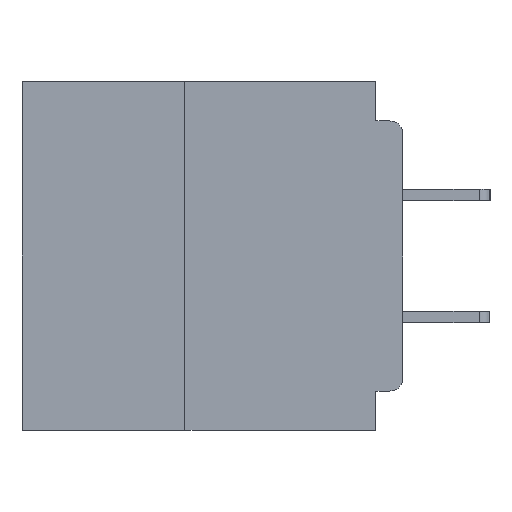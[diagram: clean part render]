
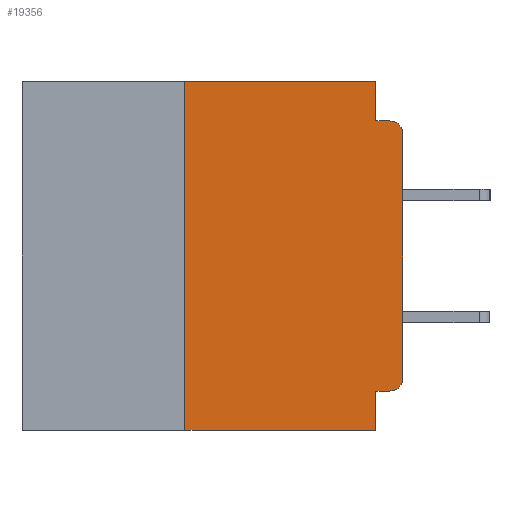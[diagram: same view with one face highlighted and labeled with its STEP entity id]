
A CAD part, left-side view. The second image highlights one B-rep face of the part: STEP entity #19356.
In plain terms, the highlighted planar face has unit normal (-1, 0, 0).
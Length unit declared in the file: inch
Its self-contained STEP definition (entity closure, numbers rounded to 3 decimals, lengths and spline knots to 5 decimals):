
#174 = ORIENTED_EDGE ( 'NONE', *, *, #10337, .T. ) ;
#470 = EDGE_CURVE ( 'NONE', #36528, #20524, #12697, .T. ) ;
#1134 = CARTESIAN_POINT ( 'NONE',  ( 0., 0.015, -0.045 ) ) ;
#1625 = CARTESIAN_POINT ( 'NONE',  ( 0., 0.031, -0.045 ) ) ;
#1760 = CARTESIAN_POINT ( 'NONE',  ( 0., 0.031, -0.355 ) ) ;
#1807 = FACE_OUTER_BOUND ( 'NONE', #8016, .T. ) ;
#3209 = CARTESIAN_POINT ( 'NONE',  ( 0., 0.031, 0. ) ) ;
#5400 = ORIENTED_EDGE ( 'NONE', *, *, #17535, .T. ) ;
#6367 = CARTESIAN_POINT ( 'NONE',  ( 0., 0.031, 0. ) ) ;
#7665 = CARTESIAN_POINT ( 'NONE',  ( 0., 0., -0.355 ) ) ;
#7924 = LINE ( 'NONE', #15533, #16364 ) ;
#8009 = VERTEX_POINT ( 'NONE', #31164 ) ;
#8016 = EDGE_LOOP ( 'NONE', ( #5400, #14799, #31670, #36529, #31976, #8084, #174, #28848, #18778, #25983 ) ) ;
#8084 = ORIENTED_EDGE ( 'NONE', *, *, #35303, .F. ) ;
#8410 = LINE ( 'NONE', #25826, #24354 ) ;
#10337 = EDGE_CURVE ( 'NONE', #20611, #20431, #35712, .T. ) ;
#11390 = VERTEX_POINT ( 'NONE', #20219 ) ;
#11866 = AXIS2_PLACEMENT_3D ( 'NONE', #40517, #15245, #37499 ) ;
#12067 = PLANE ( 'NONE',  #11866 ) ;
#12697 = LINE ( 'NONE', #6367, #28659 ) ;
#13450 = VERTEX_POINT ( 'NONE', #1134 ) ;
#13502 = DIRECTION ( 'NONE',  ( -1., 0., 0. ) ) ;
#13911 = EDGE_CURVE ( 'NONE', #20524, #13450, #8410, .T. ) ;
#14355 = DIRECTION ( 'NONE',  ( -1., 0., 0. ) ) ;
#14693 = CIRCLE ( 'NONE', #40080, 0.015 ) ;
#14799 = ORIENTED_EDGE ( 'NONE', *, *, #20332, .T. ) ;
#14854 = CARTESIAN_POINT ( 'NONE',  ( 0., 0., -0.34 ) ) ;
#15245 = DIRECTION ( 'NONE',  ( 1., 0., 0. ) ) ;
#15533 = CARTESIAN_POINT ( 'NONE',  ( 0., 0.031, -0.4 ) ) ;
#16364 = VECTOR ( 'NONE', #18724, 39.37008 ) ;
#16363 = CARTESIAN_POINT ( 'NONE',  ( 0., 0.25, -0.4 ) ) ;
#17535 = EDGE_CURVE ( 'NONE', #23939, #8009, #25613, .T. ) ;
#17722 = CIRCLE ( 'NONE', #21755, 0.015 ) ;
#18065 = CARTESIAN_POINT ( 'NONE',  ( 0., 0.25, -0.4 ) ) ;
#18724 = DIRECTION ( 'NONE',  ( 0., 0., -1. ) ) ;
#18776 = VECTOR ( 'NONE', #21428, 39.37008 ) ;
#18778 = ORIENTED_EDGE ( 'NONE', *, *, #38809, .F. ) ;
#19356 = ADVANCED_FACE ( 'NONE', ( #1807 ), #12067, .F. ) ;
#19563 = DIRECTION ( 'NONE',  ( 0., 0., 1. ) ) ;
#19798 = EDGE_CURVE ( 'NONE', #35389, #23939, #17722, .T. ) ;
#19962 = CARTESIAN_POINT ( 'NONE',  ( 0., 0.015, -0.355 ) ) ;
#19977 = LINE ( 'NONE', #24736, #22011 ) ;
#20219 = CARTESIAN_POINT ( 'NONE',  ( 0., 0.25, 0. ) ) ;
#20332 = EDGE_CURVE ( 'NONE', #8009, #13450, #14693, .T. ) ;
#20431 = VERTEX_POINT ( 'NONE', #23552 ) ;
#20524 = VERTEX_POINT ( 'NONE', #1625 ) ;
#20584 = VECTOR ( 'NONE', #23535, 39.37008 ) ;
#20611 = VERTEX_POINT ( 'NONE', #18065 ) ;
#21428 = DIRECTION ( 'NONE',  ( 0., -1., 0. ) ) ;
#21522 = CARTESIAN_POINT ( 'NONE',  ( 0., 0., 0. ) ) ;
#21755 = AXIS2_PLACEMENT_3D ( 'NONE', #33475, #14355, #36632 ) ;
#22011 = VECTOR ( 'NONE', #27947, 39.37008 ) ;
#23535 = DIRECTION ( 'NONE',  ( 0., 1., 0. ) ) ;
#23552 = CARTESIAN_POINT ( 'NONE',  ( 0., 0.031, -0.4 ) ) ;
#23939 = VERTEX_POINT ( 'NONE', #14854 ) ;
#24354 = VECTOR ( 'NONE', #32242, 39.37008 ) ;
#24736 = CARTESIAN_POINT ( 'NONE',  ( 0., 0.437, 0. ) ) ;
#25613 = LINE ( 'NONE', #21522, #38490 ) ;
#25826 = CARTESIAN_POINT ( 'NONE',  ( 0., 0., -0.045 ) ) ;
#25983 = ORIENTED_EDGE ( 'NONE', *, *, #19798, .T. ) ;
#26342 = LINE ( 'NONE', #16363, #33807 ) ;
#27947 = DIRECTION ( 'NONE',  ( 0., -1., 0. ) ) ;
#28659 = VECTOR ( 'NONE', #35020, 39.37008 ) ;
#28848 = ORIENTED_EDGE ( 'NONE', *, *, #35168, .F. ) ;
#30076 = LINE ( 'NONE', #7665, #20584 ) ;
#30776 = VERTEX_POINT ( 'NONE', #1760 ) ;
#31164 = CARTESIAN_POINT ( 'NONE',  ( 0., 0., -0.06 ) ) ;
#31670 = ORIENTED_EDGE ( 'NONE', *, *, #13911, .F. ) ;
#31976 = ORIENTED_EDGE ( 'NONE', *, *, #32882, .F. ) ;
#32242 = DIRECTION ( 'NONE',  ( 0., -1., 0. ) ) ;
#32614 = CARTESIAN_POINT ( 'NONE',  ( 0., 0.015, -0.06 ) ) ;
#32882 = EDGE_CURVE ( 'NONE', #11390, #36528, #19977, .T. ) ;
#33475 = CARTESIAN_POINT ( 'NONE',  ( 0., 0.015, -0.34 ) ) ;
#33807 = VECTOR ( 'NONE', #19563, 39.37008 ) ;
#35020 = DIRECTION ( 'NONE',  ( 0., 0., -1. ) ) ;
#35168 = EDGE_CURVE ( 'NONE', #30776, #20431, #7924, .T. ) ;
#35303 = EDGE_CURVE ( 'NONE', #20611, #11390, #26342, .T. ) ;
#35389 = VERTEX_POINT ( 'NONE', #19962 ) ;
#35712 = LINE ( 'NONE', #37264, #18776 ) ;
#35770 = DIRECTION ( 'NONE',  ( 0., 0., -1. ) ) ;
#36528 = VERTEX_POINT ( 'NONE', #3209 ) ;
#36529 = ORIENTED_EDGE ( 'NONE', *, *, #470, .F. ) ;
#36632 = DIRECTION ( 'NONE',  ( 0., 0., -1. ) ) ;
#37264 = CARTESIAN_POINT ( 'NONE',  ( 0., 0.437, -0.4 ) ) ;
#37499 = DIRECTION ( 'NONE',  ( 0., 0., -1. ) ) ;
#38490 = VECTOR ( 'NONE', #40508, 39.37008 ) ;
#38809 = EDGE_CURVE ( 'NONE', #35389, #30776, #30076, .T. ) ;
#40080 = AXIS2_PLACEMENT_3D ( 'NONE', #32614, #13502, #35770 ) ;
#40508 = DIRECTION ( 'NONE',  ( 0., 0., 1. ) ) ;
#40517 = CARTESIAN_POINT ( 'NONE',  ( 0., 0.437, 0. ) ) ;
